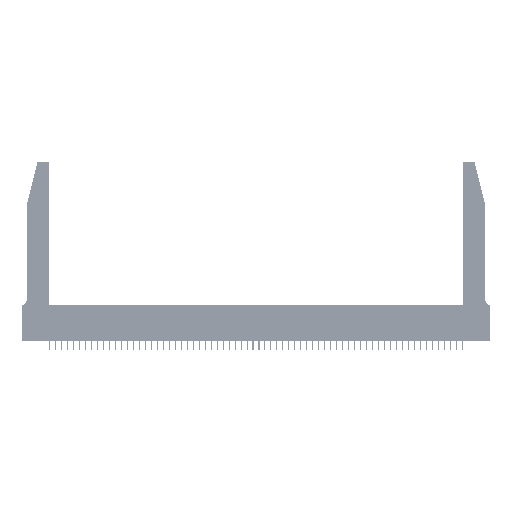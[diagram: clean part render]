
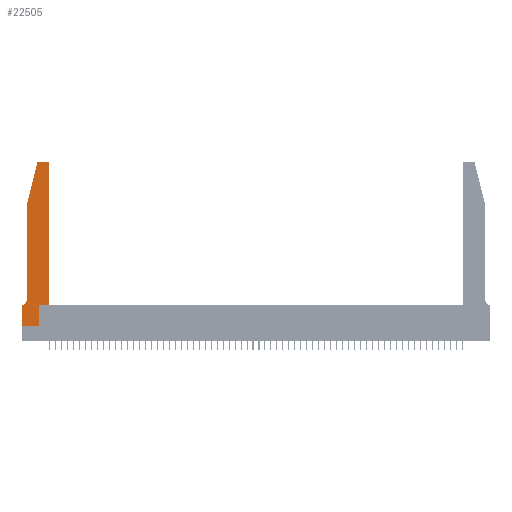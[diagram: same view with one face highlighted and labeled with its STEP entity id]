
A CAD part, top view. The second image highlights one B-rep face of the part: STEP entity #22505.
In plain terms, the highlighted planar face has unit normal (0, 0, 1).
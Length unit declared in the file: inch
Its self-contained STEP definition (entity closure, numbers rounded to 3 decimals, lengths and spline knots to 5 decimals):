
#245 = DIRECTION ( 'NONE',  ( 0., 0., 1. ) ) ;
#369 = DIRECTION ( 'NONE',  ( 0., 1., 0. ) ) ;
#1339 = DIRECTION ( 'NONE',  ( 0., -1., 0. ) ) ;
#1947 = ORIENTED_EDGE ( 'NONE', *, *, #27773, .T. ) ;
#2457 = EDGE_CURVE ( 'NONE', #46212, #20641, #45856, .T. ) ;
#2814 = CARTESIAN_POINT ( 'NONE',  ( 0.4505, 0.35, 0.37 ) ) ;
#4745 = LINE ( 'NONE', #17533, #49415 ) ;
#4810 = CARTESIAN_POINT ( 'NONE',  ( 0.2865, 0., 0.37 ) ) ;
#4839 = EDGE_CURVE ( 'NONE', #51096, #27106, #46897, .T. ) ;
#4872 = CARTESIAN_POINT ( 'NONE',  ( 0.2605, 2.75, 0.37 ) ) ;
#5263 = EDGE_CURVE ( 'NONE', #10727, #46212, #20429, .T. ) ;
#5362 = EDGE_CURVE ( 'NONE', #27106, #45383, #38736, .T. ) ;
#5777 = DIRECTION ( 'NONE',  ( -1., 0., 0. ) ) ;
#5834 = LINE ( 'NONE', #4872, #51851 ) ;
#5961 = VECTOR ( 'NONE', #43732, 39.37008 ) ;
#6965 = CARTESIAN_POINT ( 'NONE',  ( 0.284, 2.72, 0.37 ) ) ;
#9032 = EDGE_CURVE ( 'NONE', #20641, #23034, #17151, .T. ) ;
#9668 = DIRECTION ( 'NONE',  ( 0., -1., 0. ) ) ;
#9940 = ORIENTED_EDGE ( 'NONE', *, *, #39119, .T. ) ;
#10148 = CARTESIAN_POINT ( 'NONE',  ( 0.0055, 0.42, 0.37 ) ) ;
#10727 = VERTEX_POINT ( 'NONE', #39640 ) ;
#11349 = VECTOR ( 'NONE', #35788, 39.37008 ) ;
#12952 = VECTOR ( 'NONE', #40937, 39.37008 ) ;
#13352 = AXIS2_PLACEMENT_3D ( 'NONE', #23622, #32305, #49745 ) ;
#15088 = CARTESIAN_POINT ( 'NONE',  ( 0.0055, 0.35, 0.37 ) ) ;
#15233 = AXIS2_PLACEMENT_3D ( 'NONE', #6965, #37396, #33395 ) ;
#15827 = EDGE_CURVE ( 'NONE', #23034, #16385, #26238, .T. ) ;
#16178 = ORIENTED_EDGE ( 'NONE', *, *, #5263, .T. ) ;
#16385 = VERTEX_POINT ( 'NONE', #4810 ) ;
#17151 = LINE ( 'NONE', #18341, #27291 ) ;
#17225 = CARTESIAN_POINT ( 'NONE',  ( 0.4205, 2.72, 0.37 ) ) ;
#17533 = CARTESIAN_POINT ( 'NONE',  ( 0.2865, 0.35, 0.37 ) ) ;
#18306 = EDGE_LOOP ( 'NONE', ( #1947, #9940, #26045, #25935, #16178, #49952, #36072, #50559, #49996, #35642, #18720, #37640 ) ) ;
#18341 = CARTESIAN_POINT ( 'NONE',  ( 0., 0., 0.37 ) ) ;
#18617 = CIRCLE ( 'NONE', #15233, 0.03 ) ;
#18720 = ORIENTED_EDGE ( 'NONE', *, *, #5362, .T. ) ;
#19702 = CIRCLE ( 'NONE', #26295, 0.03 ) ;
#20429 = CIRCLE ( 'NONE', #36054, 0.07 ) ;
#20641 = VERTEX_POINT ( 'NONE', #32123 ) ;
#21629 = CARTESIAN_POINT ( 'NONE',  ( 0.4505, 2.72, 0.37 ) ) ;
#22505 = ADVANCED_FACE ( 'NONE', ( #44255 ), #31753, .T. ) ;
#23034 = VERTEX_POINT ( 'NONE', #55511 ) ;
#23622 = CARTESIAN_POINT ( 'NONE',  ( 0., 0.35, 0.37 ) ) ;
#24100 = CARTESIAN_POINT ( 'NONE',  ( 0.4505, 0.35, 0.37 ) ) ;
#25384 = VECTOR ( 'NONE', #55220, 39.37008 ) ;
#25715 = EDGE_CURVE ( 'NONE', #16385, #51096, #4745, .T. ) ;
#25935 = ORIENTED_EDGE ( 'NONE', *, *, #46084, .T. ) ;
#26045 = ORIENTED_EDGE ( 'NONE', *, *, #29097, .T. ) ;
#26238 = LINE ( 'NONE', #43912, #5961 ) ;
#26295 = AXIS2_PLACEMENT_3D ( 'NONE', #17225, #245, #47704 ) ;
#27106 = VERTEX_POINT ( 'NONE', #38980 ) ;
#27291 = VECTOR ( 'NONE', #1339, 39.37008 ) ;
#27773 = EDGE_CURVE ( 'NONE', #38835, #46048, #5834, .T. ) ;
#28701 = VECTOR ( 'NONE', #9668, 39.37008 ) ;
#29097 = EDGE_CURVE ( 'NONE', #38653, #34304, #53086, .T. ) ;
#31243 = CARTESIAN_POINT ( 'NONE',  ( 0.0755, 0.35, 0.37 ) ) ;
#31753 = PLANE ( 'NONE',  #13352 ) ;
#32123 = CARTESIAN_POINT ( 'NONE',  ( 0., 0.35, 0.37 ) ) ;
#32305 = DIRECTION ( 'NONE',  ( 0., 0., 1. ) ) ;
#32920 = CARTESIAN_POINT ( 'NONE',  ( 0.0755, 2., 0.37 ) ) ;
#33395 = DIRECTION ( 'NONE',  ( 1., 0., 0. ) ) ;
#34304 = VERTEX_POINT ( 'NONE', #32920 ) ;
#35509 = EDGE_CURVE ( 'NONE', #45383, #38835, #19702, .T. ) ;
#35642 = ORIENTED_EDGE ( 'NONE', *, *, #4839, .T. ) ;
#35728 = CARTESIAN_POINT ( 'NONE',  ( 0.284, 2.75, 0.37 ) ) ;
#35788 = DIRECTION ( 'NONE',  ( -1., 0., 0. ) ) ;
#36054 = AXIS2_PLACEMENT_3D ( 'NONE', #10148, #40193, #5777 ) ;
#36072 = ORIENTED_EDGE ( 'NONE', *, *, #9032, .T. ) ;
#37396 = DIRECTION ( 'NONE',  ( 0., 0., 1. ) ) ;
#37640 = ORIENTED_EDGE ( 'NONE', *, *, #35509, .T. ) ;
#37815 = CARTESIAN_POINT ( 'NONE',  ( 0.0755, 2., 0.37 ) ) ;
#38653 = VERTEX_POINT ( 'NONE', #47117 ) ;
#38736 = LINE ( 'NONE', #24100, #12952 ) ;
#38835 = VERTEX_POINT ( 'NONE', #40264 ) ;
#38980 = CARTESIAN_POINT ( 'NONE',  ( 0.4505, 0.35, 0.37 ) ) ;
#39119 = EDGE_CURVE ( 'NONE', #46048, #38653, #18617, .T. ) ;
#39640 = CARTESIAN_POINT ( 'NONE',  ( 0.0755, 0.42, 0.37 ) ) ;
#40193 = DIRECTION ( 'NONE',  ( 0., 0., -1. ) ) ;
#40264 = CARTESIAN_POINT ( 'NONE',  ( 0.4205, 2.75, 0.37 ) ) ;
#40923 = LINE ( 'NONE', #48798, #28701 ) ;
#40937 = DIRECTION ( 'NONE',  ( 0., 1., 0. ) ) ;
#43732 = DIRECTION ( 'NONE',  ( 1., 0., 0. ) ) ;
#43912 = CARTESIAN_POINT ( 'NONE',  ( 0., 0., 0.37 ) ) ;
#44255 = FACE_OUTER_BOUND ( 'NONE', #18306, .T. ) ;
#45383 = VERTEX_POINT ( 'NONE', #21629 ) ;
#45856 = LINE ( 'NONE', #31243, #11349 ) ;
#46048 = VERTEX_POINT ( 'NONE', #35728 ) ;
#46084 = EDGE_CURVE ( 'NONE', #34304, #10727, #40923, .T. ) ;
#46212 = VERTEX_POINT ( 'NONE', #15088 ) ;
#46897 = LINE ( 'NONE', #2814, #48891 ) ;
#47117 = CARTESIAN_POINT ( 'NONE',  ( 0.25487, 2.72718, 0.37 ) ) ;
#47704 = DIRECTION ( 'NONE',  ( 1., 0., 0. ) ) ;
#48019 = DIRECTION ( 'NONE',  ( -1., 0., 0. ) ) ;
#48798 = CARTESIAN_POINT ( 'NONE',  ( 0.0755, 2., 0.37 ) ) ;
#48891 = VECTOR ( 'NONE', #54993, 39.37008 ) ;
#49415 = VECTOR ( 'NONE', #369, 39.37008 ) ;
#49745 = DIRECTION ( 'NONE',  ( 1., 0., 0. ) ) ;
#49952 = ORIENTED_EDGE ( 'NONE', *, *, #2457, .T. ) ;
#49996 = ORIENTED_EDGE ( 'NONE', *, *, #25715, .T. ) ;
#50559 = ORIENTED_EDGE ( 'NONE', *, *, #15827, .T. ) ;
#51096 = VERTEX_POINT ( 'NONE', #53006 ) ;
#51851 = VECTOR ( 'NONE', #48019, 39.37008 ) ;
#53006 = CARTESIAN_POINT ( 'NONE',  ( 0.2865, 0.35, 0.37 ) ) ;
#53086 = LINE ( 'NONE', #37815, #25384 ) ;
#54993 = DIRECTION ( 'NONE',  ( 1., 0., 0. ) ) ;
#55220 = DIRECTION ( 'NONE',  ( -0.239, -0.971, 0. ) ) ;
#55511 = CARTESIAN_POINT ( 'NONE',  ( 0., 0., 0.37 ) ) ;
